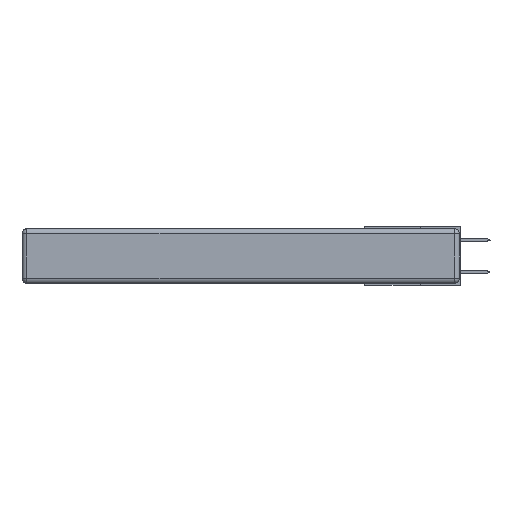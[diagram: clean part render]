
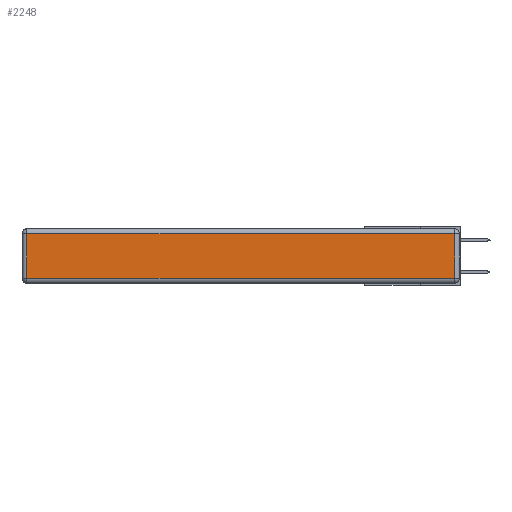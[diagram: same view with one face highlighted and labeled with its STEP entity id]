
A CAD part, left-side view. The second image highlights one B-rep face of the part: STEP entity #2248.
In plain terms, the highlighted planar face has unit normal (-1, 0, 0).
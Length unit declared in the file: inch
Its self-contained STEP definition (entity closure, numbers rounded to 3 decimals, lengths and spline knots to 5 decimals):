
#1349 = AXIS2_PLACEMENT_3D ( 'NONE', #13647, #9161, #15112 ) ;
#1532 = PLANE ( 'NONE',  #1349 ) ;
#2046 = VECTOR ( 'NONE', #9563, 39.37008 ) ;
#2248 = ADVANCED_FACE ( 'NONE', ( #3727 ), #1532, .T. ) ;
#2299 = EDGE_LOOP ( 'NONE', ( #15718, #11717, #4666, #9445 ) ) ;
#3727 = FACE_OUTER_BOUND ( 'NONE', #2299, .T. ) ;
#4518 = CARTESIAN_POINT ( 'NONE',  ( 0., 0., -0.313 ) ) ;
#4666 = ORIENTED_EDGE ( 'NONE', *, *, #18481, .T. ) ;
#5040 = VERTEX_POINT ( 'NONE', #10787 ) ;
#5286 = LINE ( 'NONE', #11051, #2046 ) ;
#6677 = LINE ( 'NONE', #9198, #19063 ) ;
#7206 = CARTESIAN_POINT ( 'NONE',  ( 0., 2.72, -0.03 ) ) ;
#7364 = DIRECTION ( 'NONE',  ( 0., -1., 0. ) ) ;
#7884 = DIRECTION ( 'NONE',  ( 0., 1., 0. ) ) ;
#9161 = DIRECTION ( 'NONE',  ( -1., 0., 0. ) ) ;
#9198 = CARTESIAN_POINT ( 'NONE',  ( 0., 2.75, -0.03 ) ) ;
#9368 = VERTEX_POINT ( 'NONE', #10151 ) ;
#9445 = ORIENTED_EDGE ( 'NONE', *, *, #9719, .T. ) ;
#9563 = DIRECTION ( 'NONE',  ( 0., 0., -1. ) ) ;
#9719 = EDGE_CURVE ( 'NONE', #19046, #5040, #5286, .T. ) ;
#10151 = CARTESIAN_POINT ( 'NONE',  ( 0., 0.03, -0.313 ) ) ;
#10275 = DIRECTION ( 'NONE',  ( 0., 0., 1. ) ) ;
#10787 = CARTESIAN_POINT ( 'NONE',  ( 0., 2.72, -0.313 ) ) ;
#11051 = CARTESIAN_POINT ( 'NONE',  ( 0., 2.72, -0.343 ) ) ;
#11701 = EDGE_CURVE ( 'NONE', #9368, #17321, #15579, .T. ) ;
#11717 = ORIENTED_EDGE ( 'NONE', *, *, #11701, .T. ) ;
#12024 = EDGE_CURVE ( 'NONE', #5040, #9368, #17225, .T. ) ;
#13041 = VECTOR ( 'NONE', #7364, 39.37008 ) ;
#13300 = CARTESIAN_POINT ( 'NONE',  ( 0., 0.03, -0.343 ) ) ;
#13647 = CARTESIAN_POINT ( 'NONE',  ( 0., 0., -0.343 ) ) ;
#15112 = DIRECTION ( 'NONE',  ( 0., 0., 1. ) ) ;
#15579 = LINE ( 'NONE', #13300, #17959 ) ;
#15718 = ORIENTED_EDGE ( 'NONE', *, *, #12024, .T. ) ;
#17127 = CARTESIAN_POINT ( 'NONE',  ( 0., 0.03, -0.03 ) ) ;
#17225 = LINE ( 'NONE', #4518, #13041 ) ;
#17321 = VERTEX_POINT ( 'NONE', #17127 ) ;
#17959 = VECTOR ( 'NONE', #10275, 39.37008 ) ;
#18481 = EDGE_CURVE ( 'NONE', #17321, #19046, #6677, .T. ) ;
#19046 = VERTEX_POINT ( 'NONE', #7206 ) ;
#19063 = VECTOR ( 'NONE', #7884, 39.37008 ) ;
